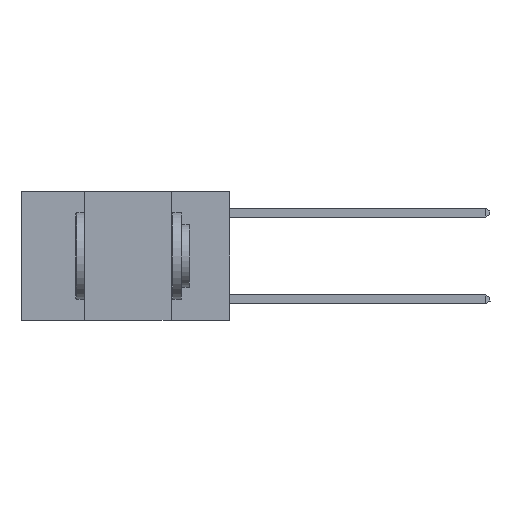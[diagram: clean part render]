
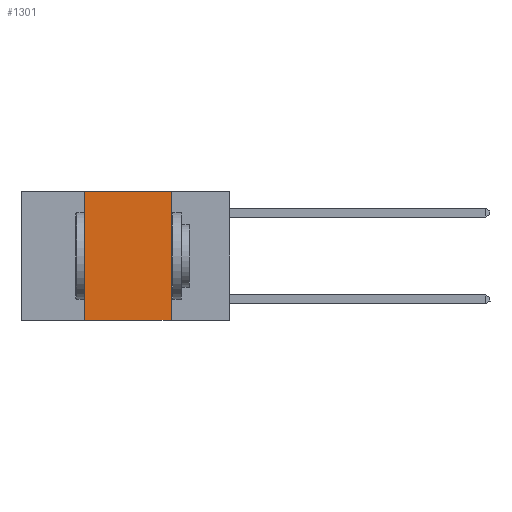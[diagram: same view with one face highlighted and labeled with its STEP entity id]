
A CAD part, left-side view. The second image highlights one B-rep face of the part: STEP entity #1301.
In plain terms, the highlighted planar face has unit normal (-1, 0, 0).
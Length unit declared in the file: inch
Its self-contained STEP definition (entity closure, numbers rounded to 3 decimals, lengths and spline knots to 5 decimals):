
#334 = AXIS2_PLACEMENT_3D ( 'NONE', #10830, #10509, #10483 ) ;
#719 = ORIENTED_EDGE ( 'NONE', *, *, #5558, .T. ) ;
#1301 = ADVANCED_FACE ( 'NONE', ( #1454 ), #10644, .F. ) ;
#1454 = FACE_OUTER_BOUND ( 'NONE', #8563, .T. ) ;
#2434 = CARTESIAN_POINT ( 'NONE',  ( 0., 0.42, 0. ) ) ;
#3822 = VECTOR ( 'NONE', #12130, 39.37008 ) ;
#4319 = VERTEX_POINT ( 'NONE', #18073 ) ;
#5280 = VECTOR ( 'NONE', #18140, 39.37008 ) ;
#5558 = EDGE_CURVE ( 'NONE', #4319, #13926, #19314, .T. ) ;
#5885 = VERTEX_POINT ( 'NONE', #2434 ) ;
#6788 = EDGE_CURVE ( 'NONE', #4319, #5885, #8738, .T. ) ;
#7198 = CARTESIAN_POINT ( 'NONE',  ( 0., 0.6, 0. ) ) ;
#8039 = CARTESIAN_POINT ( 'NONE',  ( 0., 0.17, 0. ) ) ;
#8563 = EDGE_LOOP ( 'NONE', ( #9388, #14258, #19612, #719 ) ) ;
#8738 = LINE ( 'NONE', #19340, #3822 ) ;
#9287 = EDGE_CURVE ( 'NONE', #22823, #13926, #19421, .T. ) ;
#9388 = ORIENTED_EDGE ( 'NONE', *, *, #9287, .F. ) ;
#10483 = DIRECTION ( 'NONE',  ( 0., 0., -1. ) ) ;
#10509 = DIRECTION ( 'NONE',  ( 1., 0., 0. ) ) ;
#10644 = PLANE ( 'NONE',  #334 ) ;
#10684 = CARTESIAN_POINT ( 'NONE',  ( 0., 0.17, -0.37 ) ) ;
#10817 = VECTOR ( 'NONE', #23442, 39.37008 ) ;
#10830 = CARTESIAN_POINT ( 'NONE',  ( 0., 0.6, 0. ) ) ;
#12088 = EDGE_CURVE ( 'NONE', #5885, #22823, #14501, .T. ) ;
#12130 = DIRECTION ( 'NONE',  ( 0., 0., 1. ) ) ;
#13627 = CARTESIAN_POINT ( 'NONE',  ( 0., 0.17, 0. ) ) ;
#13926 = VERTEX_POINT ( 'NONE', #10684 ) ;
#14258 = ORIENTED_EDGE ( 'NONE', *, *, #12088, .F. ) ;
#14501 = LINE ( 'NONE', #7198, #5280 ) ;
#14637 = VECTOR ( 'NONE', #18991, 39.37008 ) ;
#15900 = CARTESIAN_POINT ( 'NONE',  ( 0., 0.6, -0.37 ) ) ;
#18073 = CARTESIAN_POINT ( 'NONE',  ( 0., 0.42, -0.37 ) ) ;
#18140 = DIRECTION ( 'NONE',  ( 0., -1., 0. ) ) ;
#18991 = DIRECTION ( 'NONE',  ( 0., 0., -1. ) ) ;
#19314 = LINE ( 'NONE', #15900, #10817 ) ;
#19340 = CARTESIAN_POINT ( 'NONE',  ( 0., 0.42, 0. ) ) ;
#19421 = LINE ( 'NONE', #13627, #14637 ) ;
#19612 = ORIENTED_EDGE ( 'NONE', *, *, #6788, .F. ) ;
#22823 = VERTEX_POINT ( 'NONE', #8039 ) ;
#23442 = DIRECTION ( 'NONE',  ( 0., -1., 0. ) ) ;
